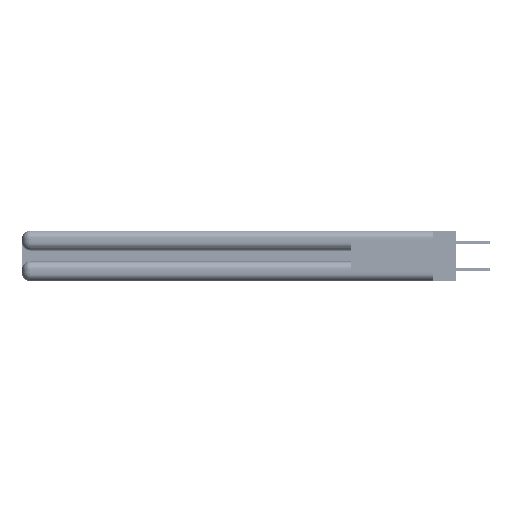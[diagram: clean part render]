
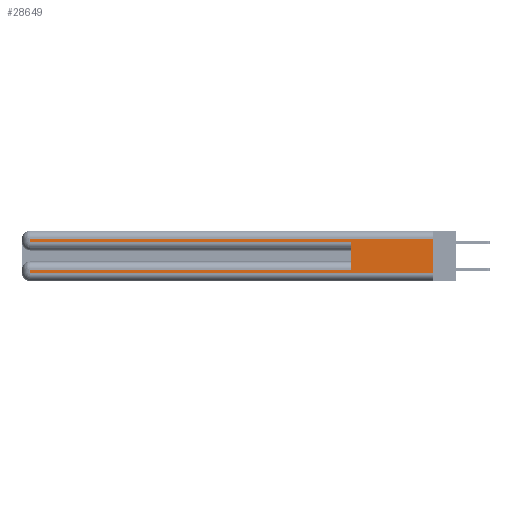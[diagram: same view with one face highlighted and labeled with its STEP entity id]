
A CAD part, left-side view. The second image highlights one B-rep face of the part: STEP entity #28649.
In plain terms, the highlighted planar face has unit normal (-1, 0, 0).
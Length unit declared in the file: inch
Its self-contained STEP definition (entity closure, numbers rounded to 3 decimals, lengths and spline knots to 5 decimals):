
#839 = EDGE_CURVE ( 'NONE', #42680, #43758, #21375, .T. ) ;
#882 = DIRECTION ( 'NONE',  ( 0., 0., -1. ) ) ;
#1933 = VECTOR ( 'NONE', #28483, 39.37008 ) ;
#2813 = ORIENTED_EDGE ( 'NONE', *, *, #839, .T. ) ;
#3997 = CARTESIAN_POINT ( 'NONE',  ( 0., 2.94, 0.285 ) ) ;
#4512 = VECTOR ( 'NONE', #7170, 39.37008 ) ;
#5668 = CARTESIAN_POINT ( 'NONE',  ( 0., 0.6, 0.285 ) ) ;
#5859 = CARTESIAN_POINT ( 'NONE',  ( 0., 0., 0.37 ) ) ;
#6013 = DIRECTION ( 'NONE',  ( 0., 0., -1. ) ) ;
#7170 = DIRECTION ( 'NONE',  ( 0., 0., -1. ) ) ;
#7263 = DIRECTION ( 'NONE',  ( 0., 0., 1. ) ) ;
#7701 = EDGE_CURVE ( 'NONE', #11193, #42680, #15131, .T. ) ;
#9020 = LINE ( 'NONE', #15290, #41444 ) ;
#9869 = DIRECTION ( 'NONE',  ( 0., 1., 0. ) ) ;
#11189 = EDGE_CURVE ( 'NONE', #28295, #23503, #39406, .T. ) ;
#11193 = VERTEX_POINT ( 'NONE', #20530 ) ;
#11672 = VECTOR ( 'NONE', #7263, 39.37008 ) ;
#11755 = ORIENTED_EDGE ( 'NONE', *, *, #23861, .T. ) ;
#12560 = PLANE ( 'NONE',  #13641 ) ;
#13079 = DIRECTION ( 'NONE',  ( 0., -1., 0. ) ) ;
#13641 = AXIS2_PLACEMENT_3D ( 'NONE', #33086, #43196, #30239 ) ;
#15131 = LINE ( 'NONE', #34985, #4512 ) ;
#15214 = LINE ( 'NONE', #21769, #1933 ) ;
#15290 = CARTESIAN_POINT ( 'NONE',  ( 0., 0., 0.285 ) ) ;
#16888 = VECTOR ( 'NONE', #9869, 39.37008 ) ;
#17071 = ORIENTED_EDGE ( 'NONE', *, *, #7701, .T. ) ;
#17848 = ORIENTED_EDGE ( 'NONE', *, *, #30069, .T. ) ;
#17922 = VECTOR ( 'NONE', #6013, 39.37008 ) ;
#18138 = FACE_OUTER_BOUND ( 'NONE', #39422, .T. ) ;
#18397 = CARTESIAN_POINT ( 'NONE',  ( 0., 0., 0.06 ) ) ;
#20480 = CARTESIAN_POINT ( 'NONE',  ( 0., 0., 0.085 ) ) ;
#20530 = CARTESIAN_POINT ( 'NONE',  ( 0., 2.94, 0.085 ) ) ;
#21375 = LINE ( 'NONE', #33444, #23520 ) ;
#21769 = CARTESIAN_POINT ( 'NONE',  ( 0., 0., 0.31 ) ) ;
#22054 = VERTEX_POINT ( 'NONE', #3997 ) ;
#23503 = VERTEX_POINT ( 'NONE', #5668 ) ;
#23520 = VECTOR ( 'NONE', #13079, 39.37008 ) ;
#23861 = EDGE_CURVE ( 'NONE', #34922, #22054, #36659, .T. ) ;
#24363 = CARTESIAN_POINT ( 'NONE',  ( 0., 0.6, 0.145 ) ) ;
#24516 = CARTESIAN_POINT ( 'NONE',  ( 0., 2.94, 0.06 ) ) ;
#28295 = VERTEX_POINT ( 'NONE', #41563 ) ;
#28483 = DIRECTION ( 'NONE',  ( 0., 1., 0. ) ) ;
#28521 = CARTESIAN_POINT ( 'NONE',  ( 0., 0., 0.31 ) ) ;
#28649 = ADVANCED_FACE ( 'NONE', ( #18138 ), #12560, .F. ) ;
#28773 = ORIENTED_EDGE ( 'NONE', *, *, #41715, .F. ) ;
#30069 = EDGE_CURVE ( 'NONE', #28295, #11193, #38198, .T. ) ;
#30239 = DIRECTION ( 'NONE',  ( 0., 0., -1. ) ) ;
#31303 = VECTOR ( 'NONE', #882, 39.37008 ) ;
#32086 = EDGE_CURVE ( 'NONE', #22054, #23503, #9020, .T. ) ;
#32499 = ORIENTED_EDGE ( 'NONE', *, *, #32086, .T. ) ;
#33086 = CARTESIAN_POINT ( 'NONE',  ( 0., 0., 0.37 ) ) ;
#33444 = CARTESIAN_POINT ( 'NONE',  ( 0., 0., 0.06 ) ) ;
#34922 = VERTEX_POINT ( 'NONE', #35870 ) ;
#34985 = CARTESIAN_POINT ( 'NONE',  ( 0., 2.94, 0.37 ) ) ;
#35536 = VERTEX_POINT ( 'NONE', #28521 ) ;
#35870 = CARTESIAN_POINT ( 'NONE',  ( 0., 2.94, 0.31 ) ) ;
#36543 = LINE ( 'NONE', #5859, #17922 ) ;
#36659 = LINE ( 'NONE', #41892, #31303 ) ;
#37518 = EDGE_CURVE ( 'NONE', #35536, #34922, #15214, .T. ) ;
#38192 = ORIENTED_EDGE ( 'NONE', *, *, #11189, .F. ) ;
#38198 = LINE ( 'NONE', #20480, #16888 ) ;
#39406 = LINE ( 'NONE', #24363, #11672 ) ;
#39422 = EDGE_LOOP ( 'NONE', ( #28773, #42496, #11755, #32499, #38192, #17848, #17071, #2813 ) ) ;
#41444 = VECTOR ( 'NONE', #42064, 39.37008 ) ;
#41563 = CARTESIAN_POINT ( 'NONE',  ( 0., 0.6, 0.085 ) ) ;
#41715 = EDGE_CURVE ( 'NONE', #35536, #43758, #36543, .T. ) ;
#41892 = CARTESIAN_POINT ( 'NONE',  ( 0., 2.94, 0.37 ) ) ;
#42064 = DIRECTION ( 'NONE',  ( 0., -1., 0. ) ) ;
#42496 = ORIENTED_EDGE ( 'NONE', *, *, #37518, .T. ) ;
#42680 = VERTEX_POINT ( 'NONE', #24516 ) ;
#43196 = DIRECTION ( 'NONE',  ( 1., 0., 0. ) ) ;
#43758 = VERTEX_POINT ( 'NONE', #18397 ) ;
